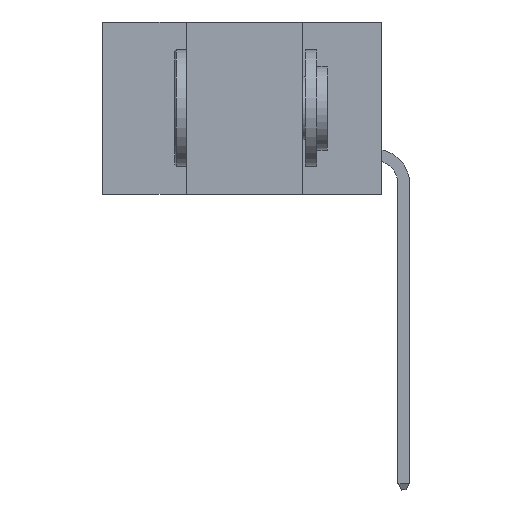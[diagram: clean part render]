
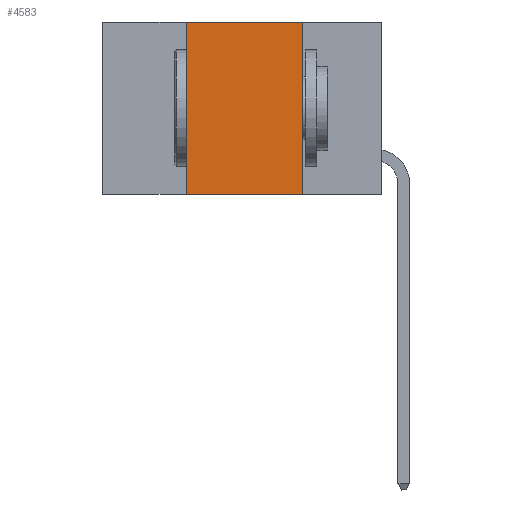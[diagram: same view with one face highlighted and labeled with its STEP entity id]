
A CAD part, left-side view. The second image highlights one B-rep face of the part: STEP entity #4583.
In plain terms, the highlighted planar face has unit normal (-1, 0, 0).
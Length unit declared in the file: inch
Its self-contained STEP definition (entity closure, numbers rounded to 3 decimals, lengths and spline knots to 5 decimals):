
#14 = VECTOR ( 'NONE', #6694, 39.37008 ) ;
#379 = LINE ( 'NONE', #1554, #6621 ) ;
#415 = DIRECTION ( 'NONE',  ( 0., -1., 0. ) ) ;
#708 = FACE_OUTER_BOUND ( 'NONE', #3992, .T. ) ;
#1472 = VECTOR ( 'NONE', #415, 39.37008 ) ;
#1554 = CARTESIAN_POINT ( 'NONE',  ( 0., 0.42, 0. ) ) ;
#2933 = LINE ( 'NONE', #6586, #1472 ) ;
#3058 = VERTEX_POINT ( 'NONE', #11962 ) ;
#3642 = ORIENTED_EDGE ( 'NONE', *, *, #5306, .F. ) ;
#3992 = EDGE_LOOP ( 'NONE', ( #3642, #12850, #5500, #12993 ) ) ;
#4257 = EDGE_CURVE ( 'NONE', #9331, #6046, #379, .T. ) ;
#4583 = ADVANCED_FACE ( 'NONE', ( #708 ), #5344, .F. ) ;
#4943 = DIRECTION ( 'NONE',  ( 0., 0., -1. ) ) ;
#4995 = AXIS2_PLACEMENT_3D ( 'NONE', #8440, #11570, #6315 ) ;
#5000 = VECTOR ( 'NONE', #4943, 39.37008 ) ;
#5306 = EDGE_CURVE ( 'NONE', #10445, #3058, #7066, .T. ) ;
#5344 = PLANE ( 'NONE',  #4995 ) ;
#5500 = ORIENTED_EDGE ( 'NONE', *, *, #4257, .F. ) ;
#6046 = VERTEX_POINT ( 'NONE', #12967 ) ;
#6315 = DIRECTION ( 'NONE',  ( 0., 0., -1. ) ) ;
#6586 = CARTESIAN_POINT ( 'NONE',  ( 0., 0.6, -0.37 ) ) ;
#6621 = VECTOR ( 'NONE', #10836, 39.37008 ) ;
#6694 = DIRECTION ( 'NONE',  ( 0., -1., 0. ) ) ;
#7066 = LINE ( 'NONE', #8964, #5000 ) ;
#8440 = CARTESIAN_POINT ( 'NONE',  ( 0., 0.6, 0. ) ) ;
#8964 = CARTESIAN_POINT ( 'NONE',  ( 0., 0.17, 0. ) ) ;
#9188 = LINE ( 'NONE', #12805, #14 ) ;
#9331 = VERTEX_POINT ( 'NONE', #9994 ) ;
#9994 = CARTESIAN_POINT ( 'NONE',  ( 0., 0.42, -0.37 ) ) ;
#10192 = CARTESIAN_POINT ( 'NONE',  ( 0., 0.17, 0. ) ) ;
#10214 = EDGE_CURVE ( 'NONE', #6046, #10445, #9188, .T. ) ;
#10445 = VERTEX_POINT ( 'NONE', #10192 ) ;
#10591 = EDGE_CURVE ( 'NONE', #9331, #3058, #2933, .T. ) ;
#10836 = DIRECTION ( 'NONE',  ( 0., 0., 1. ) ) ;
#11570 = DIRECTION ( 'NONE',  ( 1., 0., 0. ) ) ;
#11962 = CARTESIAN_POINT ( 'NONE',  ( 0., 0.17, -0.37 ) ) ;
#12805 = CARTESIAN_POINT ( 'NONE',  ( 0., 0.6, 0. ) ) ;
#12850 = ORIENTED_EDGE ( 'NONE', *, *, #10214, .F. ) ;
#12967 = CARTESIAN_POINT ( 'NONE',  ( 0., 0.42, 0. ) ) ;
#12993 = ORIENTED_EDGE ( 'NONE', *, *, #10591, .T. ) ;
